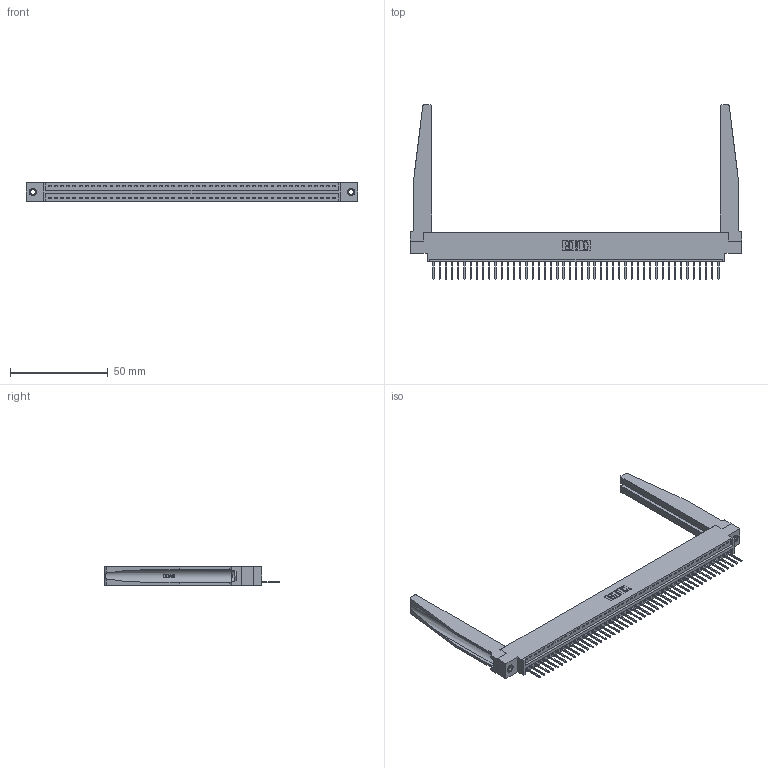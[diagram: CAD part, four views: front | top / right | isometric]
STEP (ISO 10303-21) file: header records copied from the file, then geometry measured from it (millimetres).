
FILE_DESCRIPTION (( 'STEP AP203' ), '1' );
FILE_NAME ('346-047-526-678.STEP', '2022-05-09T21:52:59', ( '' ), ( '' ), 'SwSTEP 2.0', 'SolidWorks 2020', '' );
FILE_SCHEMA (( 'CONFIG_CONTROL_DESIGN' ));
Length unit declared in the file: inch
Products named in the file (5): 345-292-001_345-293-126; 346 Part_0.170 Offset - 0.156 Dia-TH; 345-250-001_345-250-001-102; 346-047-526-678; 346-220-078_345-220-078
Assembly tree (52 placements, depth 2):
  346-047-526-678
    346 Part_0.170 Offset - 0.156 Dia-TH
    345-292-001_345-293-126  x47
    346-220-078_345-220-078  x2
    345-250-001_345-250-001-102  x2
Bounding box: 169.8 x 89.41 x 9.4 mm (x, y, z)
Volume: 7496.7 mm3; surface area: 26781.1 mm2
Topology: 51 solids, 52 shells, 3097 faces, 9257 edges, 6098 vertices
Faces by surface type: plane 2113, cylinder 932, bspline 36, cone 12, torus 4
Entity records: 33810 total; most frequent: CARTESIAN_POINT 6710, ORIENTED_EDGE 5578, DIRECTION 4897, EDGE_CURVE 2789, VECTOR 2375, LINE 2375, VERTEX_POINT 1852, AXIS2_PLACEMENT_3D 1261
